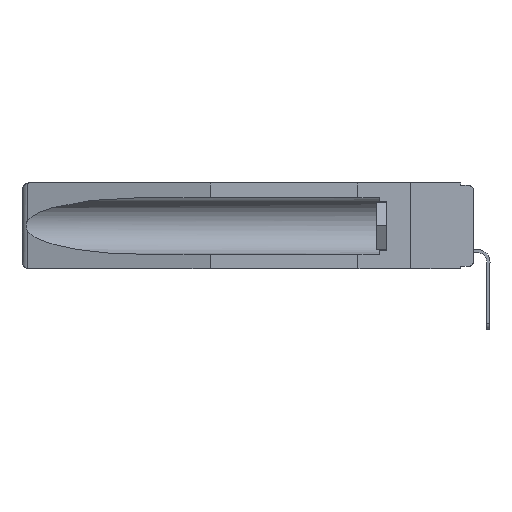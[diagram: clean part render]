
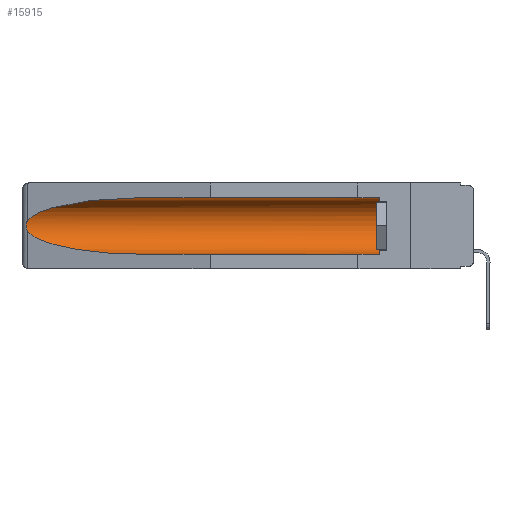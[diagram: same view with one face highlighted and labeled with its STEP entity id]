
A CAD part, left-side view. The second image highlights one B-rep face of the part: STEP entity #15915.
In plain terms, the highlighted cylindrical face has radius 2.857 mm (diameter 5.715 mm), a partial arc.
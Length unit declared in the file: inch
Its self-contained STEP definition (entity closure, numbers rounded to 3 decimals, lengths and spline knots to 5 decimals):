
#487 = ORIENTED_EDGE ( 'NONE', *, *, #10147, .T. ) ;
#684 = CARTESIAN_POINT ( 'NONE',  ( 0.26655, 1.53094, -0.18657 ) ) ;
#1794 = CARTESIAN_POINT ( 'NONE',  ( 0.155, 0.126, -0.284 ) ) ;
#1947 = CARTESIAN_POINT ( 'NONE',  ( 0.26537, 1.52718, -0.14972 ) ) ;
#1984 = B_SPLINE_CURVE_WITH_KNOTS ( 'NONE', 3,
 ( #1947, #7060, #16332, #7456, #15087, #11076, #9725, #684, #12338, #5984 ),
 .UNSPECIFIED., .F., .F.,
 ( 4, 2, 2, 2, 4 ),
 ( 0., 0.00029, 0.00058, 0.00087, 0.00117 ),
 .UNSPECIFIED. ) ;
#2022 = EDGE_CURVE ( 'NONE', #7821, #6996, #8511, .T. ) ;
#2428 = CARTESIAN_POINT ( 'NONE',  ( 0.155, -0.30754, -0.1715 ) ) ;
#2567 = DIRECTION ( 'NONE',  ( 0., 1., 0. ) ) ;
#3333 = VECTOR ( 'NONE', #2567, 39.37008 ) ;
#3682 = FACE_OUTER_BOUND ( 'NONE', #7121, .T. ) ;
#3692 = LINE ( 'NONE', #6392, #4595 ) ;
#3808 = EDGE_CURVE ( 'NONE', #12794, #7821, #1984, .T. ) ;
#4157 = CARTESIAN_POINT ( 'NONE',  ( 0.21114, 1.30732, -0.284 ) ) ;
#4595 = VECTOR ( 'NONE', #6309, 39.37008 ) ;
#4654 = CARTESIAN_POINT ( 'NONE',  ( 0.25451, 1.48313, -0.09465 ) ) ;
#4768 = EDGE_CURVE ( 'NONE', #16531, #12794, #15357, .T. ) ;
#4892 = CARTESIAN_POINT ( 'NONE',  ( 0.155, 1.07973, -0.059 ) ) ;
#5512 = DIRECTION ( 'NONE',  ( 0., -1., 0. ) ) ;
#5579 = CARTESIAN_POINT ( 'NONE',  ( 0.155, -0.30754, -0.059 ) ) ;
#5871 = EDGE_CURVE ( 'NONE', #11690, #6996, #3692, .T. ) ;
#5984 = CARTESIAN_POINT ( 'NONE',  ( 0.26537, 1.52718, -0.19328 ) ) ;
#6097 = CARTESIAN_POINT ( 'NONE',  ( 0.26537, 1.52718, -0.14972 ) ) ;
#6309 = DIRECTION ( 'NONE',  ( 0., 1., 0. ) ) ;
#6386 = AXIS2_PLACEMENT_3D ( 'NONE', #13127, #5512, #6928 ) ;
#6392 = CARTESIAN_POINT ( 'NONE',  ( 0.155, -0.30754, -0.284 ) ) ;
#6925 = CARTESIAN_POINT ( 'NONE',  ( 0.155, 1.07973, -0.284 ) ) ;
#6928 = DIRECTION ( 'NONE',  ( 0., 0., 1. ) ) ;
#6931 = CARTESIAN_POINT ( 'NONE',  ( 0.155, 1.07973, -0.059 ) ) ;
#6996 = VERTEX_POINT ( 'NONE', #7061 ) ;
#7060 = CARTESIAN_POINT ( 'NONE',  ( 0.26597, 1.52961, -0.15275 ) ) ;
#7061 = CARTESIAN_POINT ( 'NONE',  ( 0.155, 1.07973, -0.284 ) ) ;
#7121 = EDGE_LOOP ( 'NONE', ( #9445, #10503, #11049, #15840, #11780, #487 ) ) ;
#7456 = CARTESIAN_POINT ( 'NONE',  ( 0.2673, 1.5327, -0.16383 ) ) ;
#7481 = CARTESIAN_POINT ( 'NONE',  ( 0.26537, 1.52718, -0.14972 ) ) ;
#7821 = VERTEX_POINT ( 'NONE', #13232 ) ;
#8319 = CARTESIAN_POINT ( 'NONE',  ( 0.25451, 1.48313, -0.24835 ) ) ;
#8511 =( BOUNDED_CURVE ( )  B_SPLINE_CURVE ( 3, ( #13204, #8319, #4157, #6925 ),
 .UNSPECIFIED., .F., .F. ) 
 B_SPLINE_CURVE_WITH_KNOTS ( ( 4, 4 ),
 ( 0.1948, 1.5708 ),
 .UNSPECIFIED. ) 
 CURVE ( )  GEOMETRIC_REPRESENTATION_ITEM ( )  RATIONAL_B_SPLINE_CURVE ( ( 1., 0.848, 0.848, 1. ) ) 
 REPRESENTATION_ITEM ( '' )  );
#8611 = DIRECTION ( 'NONE',  ( 0., 1., 0. ) ) ;
#8780 = CYLINDRICAL_SURFACE ( 'NONE', #10401, 0.1125 ) ;
#9445 = ORIENTED_EDGE ( 'NONE', *, *, #4768, .T. ) ;
#9474 = VERTEX_POINT ( 'NONE', #10603 ) ;
#9725 = CARTESIAN_POINT ( 'NONE',  ( 0.2673, 1.53269, -0.17917 ) ) ;
#10147 = EDGE_CURVE ( 'NONE', #9474, #16531, #13273, .T. ) ;
#10401 = AXIS2_PLACEMENT_3D ( 'NONE', #2428, #8611, #13655 ) ;
#10503 = ORIENTED_EDGE ( 'NONE', *, *, #3808, .T. ) ;
#10603 = CARTESIAN_POINT ( 'NONE',  ( 0.155, 0.126, -0.059 ) ) ;
#11049 = ORIENTED_EDGE ( 'NONE', *, *, #2022, .T. ) ;
#11076 = CARTESIAN_POINT ( 'NONE',  ( 0.2675, 1.53308, -0.17534 ) ) ;
#11690 = VERTEX_POINT ( 'NONE', #1794 ) ;
#11780 = ORIENTED_EDGE ( 'NONE', *, *, #15288, .T. ) ;
#12338 = CARTESIAN_POINT ( 'NONE',  ( 0.26597, 1.5296, -0.19026 ) ) ;
#12794 = VERTEX_POINT ( 'NONE', #6097 ) ;
#13127 = CARTESIAN_POINT ( 'NONE',  ( 0.155, 0.126, -0.1715 ) ) ;
#13204 = CARTESIAN_POINT ( 'NONE',  ( 0.26537, 1.52718, -0.19328 ) ) ;
#13232 = CARTESIAN_POINT ( 'NONE',  ( 0.26537, 1.52718, -0.19328 ) ) ;
#13273 = LINE ( 'NONE', #5579, #3333 ) ;
#13589 = CIRCLE ( 'NONE', #6386, 0.1125 ) ;
#13655 = DIRECTION ( 'NONE',  ( 0., 0., 1. ) ) ;
#15087 = CARTESIAN_POINT ( 'NONE',  ( 0.2675, 1.53308, -0.16763 ) ) ;
#15288 = EDGE_CURVE ( 'NONE', #11690, #9474, #13589, .T. ) ;
#15357 =( BOUNDED_CURVE ( )  B_SPLINE_CURVE ( 3, ( #4892, #16109, #4654, #7481 ),
 .UNSPECIFIED., .F., .T. ) 
 B_SPLINE_CURVE_WITH_KNOTS ( ( 4, 4 ),
 ( 4.71239, 6.08839 ),
 .UNSPECIFIED. ) 
 CURVE ( )  GEOMETRIC_REPRESENTATION_ITEM ( )  RATIONAL_B_SPLINE_CURVE ( ( 1., 0.848, 0.848, 1. ) ) 
 REPRESENTATION_ITEM ( '' )  );
#15840 = ORIENTED_EDGE ( 'NONE', *, *, #5871, .F. ) ;
#15915 = ADVANCED_FACE ( 'NONE', ( #3682 ), #8780, .F. ) ;
#16109 = CARTESIAN_POINT ( 'NONE',  ( 0.21114, 1.30732, -0.059 ) ) ;
#16332 = CARTESIAN_POINT ( 'NONE',  ( 0.26654, 1.53092, -0.15636 ) ) ;
#16531 = VERTEX_POINT ( 'NONE', #6931 ) ;
